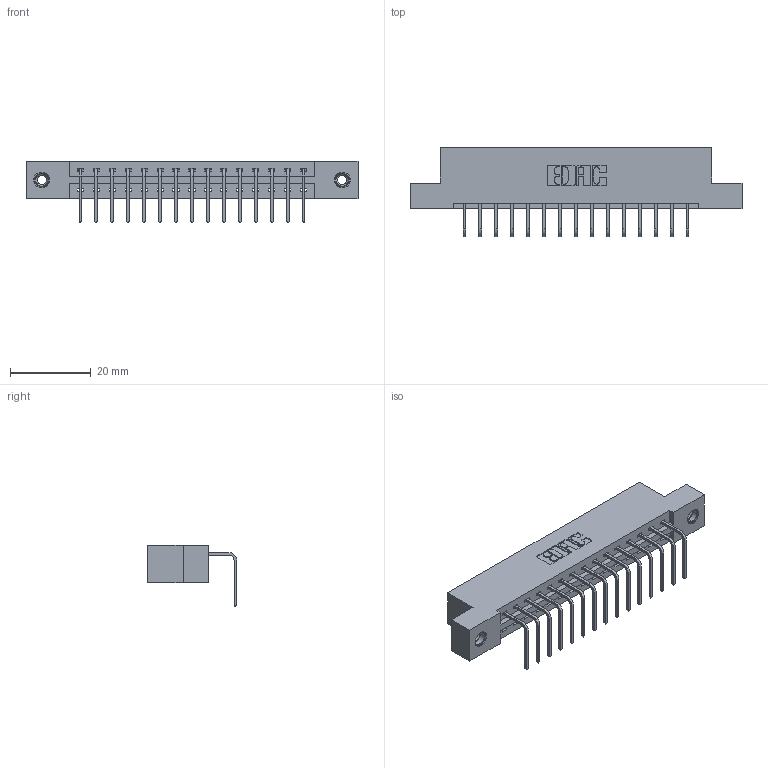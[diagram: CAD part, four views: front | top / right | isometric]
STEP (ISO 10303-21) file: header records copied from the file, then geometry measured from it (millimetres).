
FILE_DESCRIPTION (( 'STEP AP203' ), '1' );
FILE_NAME ('387-015-558-108.STEP', '2019-10-07T16:58:53', ( '' ), ( '' ), 'SwSTEP 2.0', 'SolidWorks 2016', '' );
FILE_SCHEMA (( 'CONFIG_CONTROL_DESIGN' ));
Length unit declared in the file: inch
Products named in the file (4): 345-250-001_345-250-003-102; 387-015-558-108; 337 Part_Flush Mounting Lugs - 0.156 Dia-TI; 345-292-001_558 Tail - 2
Assembly tree (18 placements, depth 2):
  387-015-558-108
    337 Part_Flush Mounting Lugs - 0.156 Dia-TI
    345-292-001_558 Tail - 2  x15
    345-250-001_345-250-003-102  x2
Bounding box: 82.45 x 22.17 x 15.37 mm (x, y, z)
Volume: 8274.7 mm3; surface area: 8737.6 mm2
Topology: 18 solids, 18 shells, 1134 faces, 3357 edges, 2210 vertices
Faces by surface type: plane 822, cylinder 296, cone 12, torus 4
Entity records: 15912 total; most frequent: CARTESIAN_POINT 2750, ORIENTED_EDGE 2694, DIRECTION 2403, EDGE_CURVE 1347, LINE 1199, VECTOR 1199, VERTEX_POINT 892, AXIS2_PLACEMENT_3D 602
